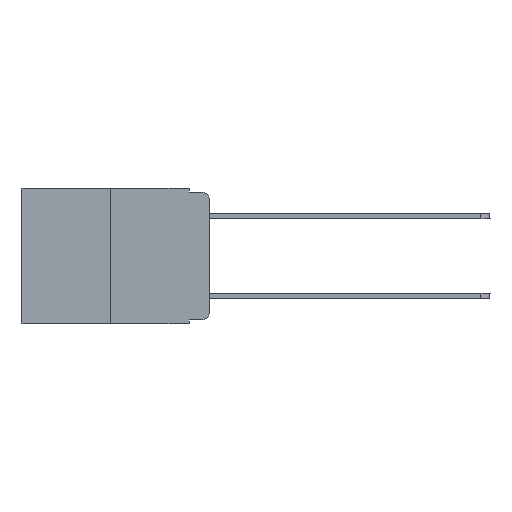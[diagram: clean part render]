
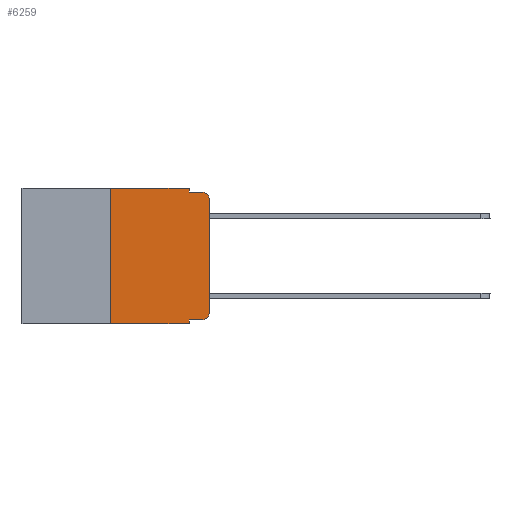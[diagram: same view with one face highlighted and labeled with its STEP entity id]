
A CAD part, left-side view. The second image highlights one B-rep face of the part: STEP entity #6259.
In plain terms, the highlighted planar face has unit normal (-1, 0, 0).
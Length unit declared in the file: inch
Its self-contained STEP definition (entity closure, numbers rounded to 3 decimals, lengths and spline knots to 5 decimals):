
#265 = DIRECTION ( 'NONE',  ( 0., 0., -1. ) ) ;
#307 = EDGE_CURVE ( 'NONE', #16233, #14076, #16396, .T. ) ;
#317 = DIRECTION ( 'NONE',  ( -1., 0., 0. ) ) ;
#1064 = ORIENTED_EDGE ( 'NONE', *, *, #307, .F. ) ;
#1189 = ORIENTED_EDGE ( 'NONE', *, *, #12614, .F. ) ;
#1325 = VECTOR ( 'NONE', #6570, 39.37008 ) ;
#1718 = AXIS2_PLACEMENT_3D ( 'NONE', #8675, #17084, #2705 ) ;
#1860 = LINE ( 'NONE', #14106, #16699 ) ;
#1890 = CARTESIAN_POINT ( 'NONE',  ( 0., 0.051, 0. ) ) ;
#1904 = EDGE_CURVE ( 'NONE', #6080, #1937, #3912, .T. ) ;
#1918 = ORIENTED_EDGE ( 'NONE', *, *, #9040, .T. ) ;
#1937 = VERTEX_POINT ( 'NONE', #13788 ) ;
#2272 = CARTESIAN_POINT ( 'NONE',  ( 0., 0.02, -0.333 ) ) ;
#2473 = AXIS2_PLACEMENT_3D ( 'NONE', #10337, #7713, #14899 ) ;
#2659 = VERTEX_POINT ( 'NONE', #6117 ) ;
#2705 = DIRECTION ( 'NONE',  ( 0., 0., -1. ) ) ;
#2707 = CARTESIAN_POINT ( 'NONE',  ( 0., 0.473, 0. ) ) ;
#3301 = ORIENTED_EDGE ( 'NONE', *, *, #18312, .F. ) ;
#3610 = VECTOR ( 'NONE', #4164, 39.37008 ) ;
#3788 = CIRCLE ( 'NONE', #1718, 0.02 ) ;
#3912 = LINE ( 'NONE', #10161, #11303 ) ;
#3948 = CARTESIAN_POINT ( 'NONE',  ( 0., 0.25, 0. ) ) ;
#4164 = DIRECTION ( 'NONE',  ( 0., -1., 0. ) ) ;
#4195 = FACE_OUTER_BOUND ( 'NONE', #18126, .T. ) ;
#4435 = VERTEX_POINT ( 'NONE', #14449 ) ;
#4491 = DIRECTION ( 'NONE',  ( 0., 0., -1. ) ) ;
#4601 = ORIENTED_EDGE ( 'NONE', *, *, #9899, .T. ) ;
#5141 = VECTOR ( 'NONE', #12915, 39.37008 ) ;
#5493 = EDGE_CURVE ( 'NONE', #16233, #16050, #7168, .T. ) ;
#5617 = CARTESIAN_POINT ( 'NONE',  ( 0., 0., 0. ) ) ;
#5950 = CARTESIAN_POINT ( 'NONE',  ( 0., 0.051, 0. ) ) ;
#5977 = CIRCLE ( 'NONE', #7420, 0.02 ) ;
#6080 = VERTEX_POINT ( 'NONE', #5950 ) ;
#6117 = CARTESIAN_POINT ( 'NONE',  ( 0., 0.25, -0.343 ) ) ;
#6259 = ADVANCED_FACE ( 'NONE', ( #4195 ), #16292, .F. ) ;
#6570 = DIRECTION ( 'NONE',  ( 0., 0., -1. ) ) ;
#6907 = VERTEX_POINT ( 'NONE', #14738 ) ;
#7168 = LINE ( 'NONE', #10359, #12059 ) ;
#7420 = AXIS2_PLACEMENT_3D ( 'NONE', #8889, #317, #265 ) ;
#7713 = DIRECTION ( 'NONE',  ( 1., 0., 0. ) ) ;
#8675 = CARTESIAN_POINT ( 'NONE',  ( 0., 0.02, -0.313 ) ) ;
#8842 = DIRECTION ( 'NONE',  ( 0., -1., 0. ) ) ;
#8889 = CARTESIAN_POINT ( 'NONE',  ( 0., 0.02, -0.03 ) ) ;
#9040 = EDGE_CURVE ( 'NONE', #2659, #14076, #12675, .T. ) ;
#9231 = LINE ( 'NONE', #5617, #14582 ) ;
#9899 = EDGE_CURVE ( 'NONE', #6907, #4435, #5977, .T. ) ;
#10161 = CARTESIAN_POINT ( 'NONE',  ( 0., 0.051, 0. ) ) ;
#10337 = CARTESIAN_POINT ( 'NONE',  ( 0., 0.473, 0. ) ) ;
#10359 = CARTESIAN_POINT ( 'NONE',  ( 0., 0.051, -0.333 ) ) ;
#10922 = EDGE_CURVE ( 'NONE', #1937, #4435, #1860, .T. ) ;
#10984 = LINE ( 'NONE', #18459, #5141 ) ;
#11263 = DIRECTION ( 'NONE',  ( 0., 0., 1. ) ) ;
#11303 = VECTOR ( 'NONE', #4491, 39.37008 ) ;
#11975 = ORIENTED_EDGE ( 'NONE', *, *, #5493, .T. ) ;
#12059 = VECTOR ( 'NONE', #8842, 39.37008 ) ;
#12272 = ORIENTED_EDGE ( 'NONE', *, *, #10922, .F. ) ;
#12474 = VECTOR ( 'NONE', #12548, 39.37008 ) ;
#12548 = DIRECTION ( 'NONE',  ( 0., -1., 0. ) ) ;
#12614 = EDGE_CURVE ( 'NONE', #17521, #6080, #17510, .T. ) ;
#12666 = EDGE_CURVE ( 'NONE', #14406, #6907, #9231, .T. ) ;
#12675 = LINE ( 'NONE', #15380, #12474 ) ;
#12911 = ORIENTED_EDGE ( 'NONE', *, *, #1904, .F. ) ;
#12915 = DIRECTION ( 'NONE',  ( 0., 0., 1. ) ) ;
#13788 = CARTESIAN_POINT ( 'NONE',  ( 0., 0.051, -0.01 ) ) ;
#14076 = VERTEX_POINT ( 'NONE', #14576 ) ;
#14106 = CARTESIAN_POINT ( 'NONE',  ( 0., 0.051, -0.01 ) ) ;
#14377 = CARTESIAN_POINT ( 'NONE',  ( 0., 0.051, -0.333 ) ) ;
#14406 = VERTEX_POINT ( 'NONE', #17449 ) ;
#14449 = CARTESIAN_POINT ( 'NONE',  ( 0., 0.02, -0.01 ) ) ;
#14576 = CARTESIAN_POINT ( 'NONE',  ( 0., 0.051, -0.343 ) ) ;
#14582 = VECTOR ( 'NONE', #11263, 39.37008 ) ;
#14738 = CARTESIAN_POINT ( 'NONE',  ( 0., 0., -0.03 ) ) ;
#14899 = DIRECTION ( 'NONE',  ( 0., 0., -1. ) ) ;
#15380 = CARTESIAN_POINT ( 'NONE',  ( 0., 0.473, -0.343 ) ) ;
#15746 = DIRECTION ( 'NONE',  ( 0., -1., 0. ) ) ;
#16050 = VERTEX_POINT ( 'NONE', #2272 ) ;
#16233 = VERTEX_POINT ( 'NONE', #14377 ) ;
#16292 = PLANE ( 'NONE',  #2473 ) ;
#16386 = ORIENTED_EDGE ( 'NONE', *, *, #12666, .T. ) ;
#16396 = LINE ( 'NONE', #1890, #1325 ) ;
#16699 = VECTOR ( 'NONE', #15746, 39.37008 ) ;
#17084 = DIRECTION ( 'NONE',  ( -1., 0., 0. ) ) ;
#17449 = CARTESIAN_POINT ( 'NONE',  ( 0., 0., -0.313 ) ) ;
#17510 = LINE ( 'NONE', #2707, #3610 ) ;
#17521 = VERTEX_POINT ( 'NONE', #3948 ) ;
#18126 = EDGE_LOOP ( 'NONE', ( #16386, #4601, #12272, #12911, #1189, #3301, #1918, #1064, #11975, #18267 ) ) ;
#18267 = ORIENTED_EDGE ( 'NONE', *, *, #18291, .T. ) ;
#18291 = EDGE_CURVE ( 'NONE', #16050, #14406, #3788, .T. ) ;
#18312 = EDGE_CURVE ( 'NONE', #2659, #17521, #10984, .T. ) ;
#18459 = CARTESIAN_POINT ( 'NONE',  ( 0., 0.25, 0. ) ) ;
